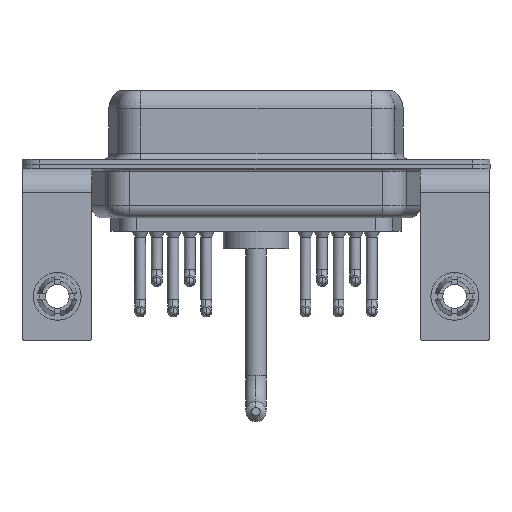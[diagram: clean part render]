
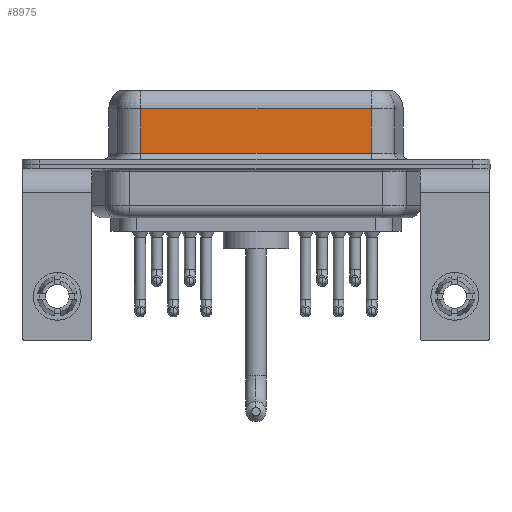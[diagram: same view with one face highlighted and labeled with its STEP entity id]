
A CAD part, front view. The second image highlights one B-rep face of the part: STEP entity #8975.
In plain terms, the highlighted planar face has unit normal (0, -1, 0).
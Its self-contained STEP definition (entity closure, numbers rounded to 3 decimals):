
#642 = EDGE_LOOP ( 'NONE', ( #9601, #19448, #14375, #13813 ) ) ;
#962 = CARTESIAN_POINT ( 'NONE',  ( 7.013, -3.95, 4.65 ) ) ;
#1060 = VECTOR ( 'NONE', #14060, 1000. ) ;
#1362 = CARTESIAN_POINT ( 'NONE',  ( 7.013, -3.95, 0.9 ) ) ;
#1410 = VERTEX_POINT ( 'NONE', #962 ) ;
#1949 = DIRECTION ( 'NONE',  ( 1., 0., 0. ) ) ;
#2369 = AXIS2_PLACEMENT_3D ( 'NONE', #17173, #7565, #4174 ) ;
#2835 = CARTESIAN_POINT ( 'NONE',  ( 26.287, -3.95, 4.65 ) ) ;
#4174 = DIRECTION ( 'NONE',  ( 0., 0., 1. ) ) ;
#4380 = FACE_OUTER_BOUND ( 'NONE', #642, .T. ) ;
#5378 = VERTEX_POINT ( 'NONE', #19268 ) ;
#5970 = CARTESIAN_POINT ( 'NONE',  ( 7.013, -3.95, 6.4 ) ) ;
#7565 = DIRECTION ( 'NONE',  ( 0., 1., 0. ) ) ;
#8907 = CARTESIAN_POINT ( 'NONE',  ( 26.287, -3.95, 6.4 ) ) ;
#8975 = ADVANCED_FACE ( 'NONE', ( #4380 ), #19067, .F. ) ;
#8980 = LINE ( 'NONE', #5970, #1060 ) ;
#9601 = ORIENTED_EDGE ( 'NONE', *, *, #19355, .F. ) ;
#9610 = EDGE_CURVE ( 'NONE', #10199, #5378, #18120, .T. ) ;
#10199 = VERTEX_POINT ( 'NONE', #1362 ) ;
#11976 = VECTOR ( 'NONE', #17424, 1000. ) ;
#12281 = EDGE_CURVE ( 'NONE', #1410, #10199, #8980, .T. ) ;
#13284 = EDGE_CURVE ( 'NONE', #14366, #1410, #19112, .T. ) ;
#13571 = LINE ( 'NONE', #8907, #19089 ) ;
#13813 = ORIENTED_EDGE ( 'NONE', *, *, #9610, .T. ) ;
#14060 = DIRECTION ( 'NONE',  ( 0., 0., -1. ) ) ;
#14366 = VERTEX_POINT ( 'NONE', #18025 ) ;
#14375 = ORIENTED_EDGE ( 'NONE', *, *, #12281, .T. ) ;
#15291 = VECTOR ( 'NONE', #1949, 1000. ) ;
#15380 = DIRECTION ( 'NONE',  ( 0., 0., -1. ) ) ;
#16536 = CARTESIAN_POINT ( 'NONE',  ( 26.287, -3.95, 0.9 ) ) ;
#17173 = CARTESIAN_POINT ( 'NONE',  ( 26.287, -3.95, 6.4 ) ) ;
#17424 = DIRECTION ( 'NONE',  ( -1., 0., 0. ) ) ;
#18025 = CARTESIAN_POINT ( 'NONE',  ( 26.287, -3.95, 4.65 ) ) ;
#18120 = LINE ( 'NONE', #16536, #15291 ) ;
#19067 = PLANE ( 'NONE',  #2369 ) ;
#19089 = VECTOR ( 'NONE', #15380, 1000. ) ;
#19112 = LINE ( 'NONE', #2835, #11976 ) ;
#19268 = CARTESIAN_POINT ( 'NONE',  ( 26.287, -3.95, 0.9 ) ) ;
#19355 = EDGE_CURVE ( 'NONE', #14366, #5378, #13571, .T. ) ;
#19448 = ORIENTED_EDGE ( 'NONE', *, *, #13284, .T. ) ;
